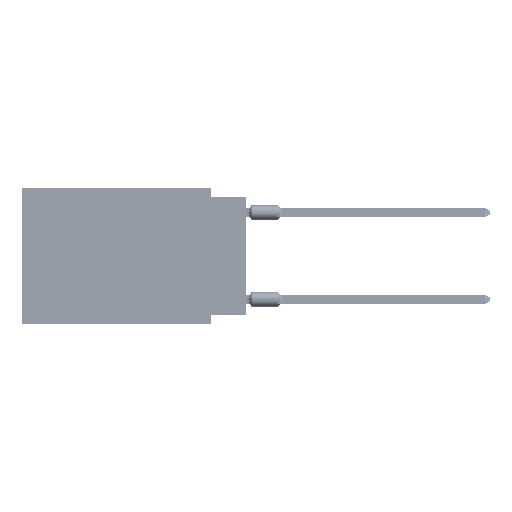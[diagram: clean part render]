
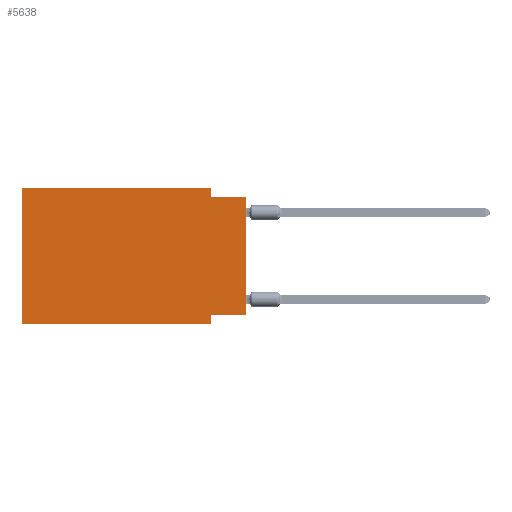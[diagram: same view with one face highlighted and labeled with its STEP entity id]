
A CAD part, left-side view. The second image highlights one B-rep face of the part: STEP entity #5638.
In plain terms, the highlighted planar face has unit normal (-1, 0, 0).
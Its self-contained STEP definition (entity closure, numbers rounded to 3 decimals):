
#505 = CARTESIAN_POINT ( 'NONE',  ( 0., 16.383, -9.906 ) ) ;
#1680 = VECTOR ( 'NONE', #56972, 1000. ) ;
#1821 = DIRECTION ( 'NONE',  ( 0., 0., 1. ) ) ;
#3329 = FACE_OUTER_BOUND ( 'NONE', #53338, .T. ) ;
#3623 = ORIENTED_EDGE ( 'NONE', *, *, #33457, .F. ) ;
#4056 = CARTESIAN_POINT ( 'NONE',  ( 0., 16.383, 0. ) ) ;
#4815 = DIRECTION ( 'NONE',  ( 0., 1., 0. ) ) ;
#4891 = VERTEX_POINT ( 'NONE', #63472 ) ;
#5638 = ADVANCED_FACE ( 'NONE', ( #3329 ), #63288, .F. ) ;
#6788 = ORIENTED_EDGE ( 'NONE', *, *, #55716, .T. ) ;
#7000 = VERTEX_POINT ( 'NONE', #26108 ) ;
#7017 = LINE ( 'NONE', #61854, #43362 ) ;
#7974 = VERTEX_POINT ( 'NONE', #35841 ) ;
#8090 = VECTOR ( 'NONE', #4815, 1000. ) ;
#11141 = EDGE_CURVE ( 'NONE', #7000, #57499, #7017, .T. ) ;
#12230 = LINE ( 'NONE', #60024, #17461 ) ;
#17461 = VECTOR ( 'NONE', #70268, 1000. ) ;
#17755 = CARTESIAN_POINT ( 'NONE',  ( 0., 0., -9.271 ) ) ;
#18516 = DIRECTION ( 'NONE',  ( 0., -1., 0. ) ) ;
#20148 = VECTOR ( 'NONE', #70576, 1000. ) ;
#24032 = LINE ( 'NONE', #17755, #8090 ) ;
#24712 = ORIENTED_EDGE ( 'NONE', *, *, #35525, .T. ) ;
#24808 = VERTEX_POINT ( 'NONE', #58144 ) ;
#26108 = CARTESIAN_POINT ( 'NONE',  ( 0., 16.383, -9.906 ) ) ;
#27240 = CARTESIAN_POINT ( 'NONE',  ( 0., 16.383, 0. ) ) ;
#27620 = EDGE_CURVE ( 'NONE', #4891, #70232, #24032, .T. ) ;
#30361 = CARTESIAN_POINT ( 'NONE',  ( 0., 2.54, -9.906 ) ) ;
#31627 = ORIENTED_EDGE ( 'NONE', *, *, #11141, .F. ) ;
#32006 = DIRECTION ( 'NONE',  ( 0., 0., -1. ) ) ;
#33108 = LINE ( 'NONE', #4056, #1680 ) ;
#33457 = EDGE_CURVE ( 'NONE', #44037, #7974, #12230, .T. ) ;
#34567 = LINE ( 'NONE', #63126, #20148 ) ;
#35525 = EDGE_CURVE ( 'NONE', #4891, #7974, #73884, .T. ) ;
#35841 = CARTESIAN_POINT ( 'NONE',  ( 0., 0., -0.635 ) ) ;
#36739 = EDGE_CURVE ( 'NONE', #24808, #44037, #34567, .T. ) ;
#38867 = ORIENTED_EDGE ( 'NONE', *, *, #44898, .F. ) ;
#42205 = CARTESIAN_POINT ( 'NONE',  ( 0., 2.54, -9.906 ) ) ;
#43362 = VECTOR ( 'NONE', #67336, 1000. ) ;
#44037 = VERTEX_POINT ( 'NONE', #45407 ) ;
#44898 = EDGE_CURVE ( 'NONE', #57499, #24808, #33108, .T. ) ;
#45356 = ORIENTED_EDGE ( 'NONE', *, *, #27620, .F. ) ;
#45407 = CARTESIAN_POINT ( 'NONE',  ( 0., 2.54, -0.635 ) ) ;
#46262 = VECTOR ( 'NONE', #18516, 1000. ) ;
#48483 = VERTEX_POINT ( 'NONE', #42205 ) ;
#48666 = LINE ( 'NONE', #505, #46262 ) ;
#50766 = DIRECTION ( 'NONE',  ( 1., 0., 0. ) ) ;
#52422 = EDGE_CURVE ( 'NONE', #70232, #48483, #60119, .T. ) ;
#53338 = EDGE_LOOP ( 'NONE', ( #24712, #3623, #61414, #38867, #31627, #6788, #55195, #45356 ) ) ;
#55195 = ORIENTED_EDGE ( 'NONE', *, *, #52422, .F. ) ;
#55716 = EDGE_CURVE ( 'NONE', #7000, #48483, #48666, .T. ) ;
#56972 = DIRECTION ( 'NONE',  ( 0., -1., 0. ) ) ;
#57499 = VERTEX_POINT ( 'NONE', #70868 ) ;
#58144 = CARTESIAN_POINT ( 'NONE',  ( 0., 2.54, 0. ) ) ;
#60024 = CARTESIAN_POINT ( 'NONE',  ( 0., 0., -0.635 ) ) ;
#60119 = LINE ( 'NONE', #30361, #71147 ) ;
#61279 = DIRECTION ( 'NONE',  ( 0., 0., -1. ) ) ;
#61414 = ORIENTED_EDGE ( 'NONE', *, *, #36739, .F. ) ;
#61854 = CARTESIAN_POINT ( 'NONE',  ( 0., 16.383, 0. ) ) ;
#63126 = CARTESIAN_POINT ( 'NONE',  ( 0., 2.54, 0. ) ) ;
#63288 = PLANE ( 'NONE',  #70366 ) ;
#63472 = CARTESIAN_POINT ( 'NONE',  ( 0., 0., -9.271 ) ) ;
#66468 = CARTESIAN_POINT ( 'NONE',  ( 0., 0., 0. ) ) ;
#67105 = CARTESIAN_POINT ( 'NONE',  ( 0., 2.54, -9.271 ) ) ;
#67336 = DIRECTION ( 'NONE',  ( 0., 0., 1. ) ) ;
#70232 = VERTEX_POINT ( 'NONE', #67105 ) ;
#70268 = DIRECTION ( 'NONE',  ( 0., -1., 0. ) ) ;
#70366 = AXIS2_PLACEMENT_3D ( 'NONE', #27240, #50766, #32006 ) ;
#70576 = DIRECTION ( 'NONE',  ( 0., 0., -1. ) ) ;
#70868 = CARTESIAN_POINT ( 'NONE',  ( 0., 16.383, 0. ) ) ;
#71147 = VECTOR ( 'NONE', #61279, 1000. ) ;
#73884 = LINE ( 'NONE', #66468, #75200 ) ;
#75200 = VECTOR ( 'NONE', #1821, 1000. ) ;
